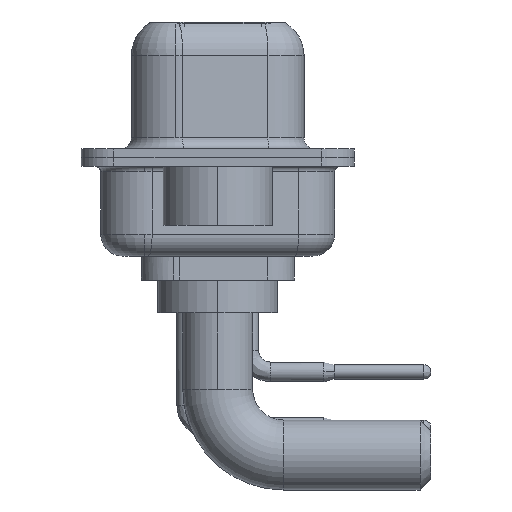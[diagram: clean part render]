
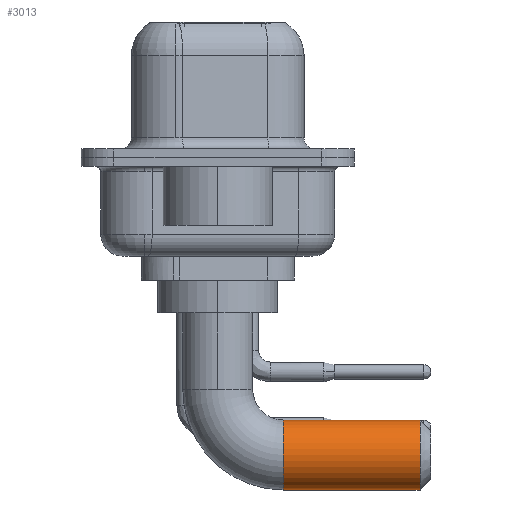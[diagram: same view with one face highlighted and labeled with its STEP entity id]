
A CAD part, left-side view. The second image highlights one B-rep face of the part: STEP entity #3013.
In plain terms, the highlighted cylindrical face has radius 1.6 mm (diameter 3.2 mm), a partial arc.
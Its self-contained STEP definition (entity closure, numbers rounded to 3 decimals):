
#307 = ORIENTED_EDGE ( 'NONE', *, *, #18518, .T. ) ;
#421 = CARTESIAN_POINT ( 'NONE',  ( 0., -9.25, -4.9 ) ) ;
#606 = CYLINDRICAL_SURFACE ( 'NONE', #1763, 1.6 ) ;
#1070 = EDGE_CURVE ( 'NONE', #11325, #4282, #4332, .T. ) ;
#1097 = DIRECTION ( 'NONE',  ( 0., -1., 0. ) ) ;
#1270 = CIRCLE ( 'NONE', #9004, 1.6 ) ;
#1763 = AXIS2_PLACEMENT_3D ( 'NONE', #13835, #1097, #9105 ) ;
#1767 = DIRECTION ( 'NONE',  ( 0., -1., 0. ) ) ;
#2071 = FACE_OUTER_BOUND ( 'NONE', #13328, .T. ) ;
#2366 = AXIS2_PLACEMENT_3D ( 'NONE', #3232, #12814, #2826 ) ;
#2826 = DIRECTION ( 'NONE',  ( 0., 0., -1. ) ) ;
#3013 = ADVANCED_FACE ( 'NONE', ( #2071 ), #606, .T. ) ;
#3232 = CARTESIAN_POINT ( 'NONE',  ( 0., -9.25, -6.5 ) ) ;
#3444 = CARTESIAN_POINT ( 'NONE',  ( 0., -3., -8.1 ) ) ;
#3772 = LINE ( 'NONE', #6819, #7075 ) ;
#3866 = ORIENTED_EDGE ( 'NONE', *, *, #5642, .T. ) ;
#4282 = VERTEX_POINT ( 'NONE', #421 ) ;
#4332 = LINE ( 'NONE', #10758, #12813 ) ;
#4916 = DIRECTION ( 'NONE',  ( -1., 0., 0. ) ) ;
#5642 = EDGE_CURVE ( 'NONE', #11325, #13213, #1270, .T. ) ;
#6819 = CARTESIAN_POINT ( 'NONE',  ( 0., -3., -8.1 ) ) ;
#7075 = VECTOR ( 'NONE', #16615, 1000. ) ;
#7517 = VERTEX_POINT ( 'NONE', #12539 ) ;
#7706 = DIRECTION ( 'NONE',  ( 0., -1., 0. ) ) ;
#9004 = AXIS2_PLACEMENT_3D ( 'NONE', #11249, #1767, #4916 ) ;
#9105 = DIRECTION ( 'NONE',  ( 0., 0., -1. ) ) ;
#10758 = CARTESIAN_POINT ( 'NONE',  ( 0., -3., -4.9 ) ) ;
#11249 = CARTESIAN_POINT ( 'NONE',  ( 0., -3., -6.5 ) ) ;
#11325 = VERTEX_POINT ( 'NONE', #12079 ) ;
#12079 = CARTESIAN_POINT ( 'NONE',  ( 0., -3., -4.9 ) ) ;
#12539 = CARTESIAN_POINT ( 'NONE',  ( 0., -9.25, -8.1 ) ) ;
#12747 = ORIENTED_EDGE ( 'NONE', *, *, #16856, .T. ) ;
#12813 = VECTOR ( 'NONE', #7706, 1000. ) ;
#12814 = DIRECTION ( 'NONE',  ( 0., 1., 0. ) ) ;
#13213 = VERTEX_POINT ( 'NONE', #3444 ) ;
#13328 = EDGE_LOOP ( 'NONE', ( #13872, #3866, #307, #12747 ) ) ;
#13835 = CARTESIAN_POINT ( 'NONE',  ( 0., -3., -6.5 ) ) ;
#13872 = ORIENTED_EDGE ( 'NONE', *, *, #1070, .F. ) ;
#14804 = CIRCLE ( 'NONE', #2366, 1.6 ) ;
#16615 = DIRECTION ( 'NONE',  ( 0., -1., 0. ) ) ;
#16856 = EDGE_CURVE ( 'NONE', #7517, #4282, #14804, .T. ) ;
#18518 = EDGE_CURVE ( 'NONE', #13213, #7517, #3772, .T. ) ;
